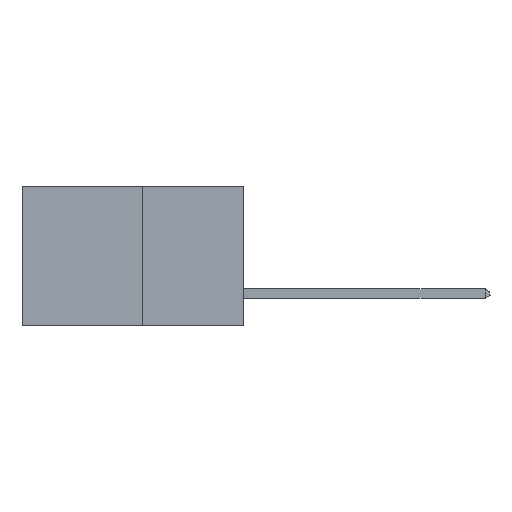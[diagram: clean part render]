
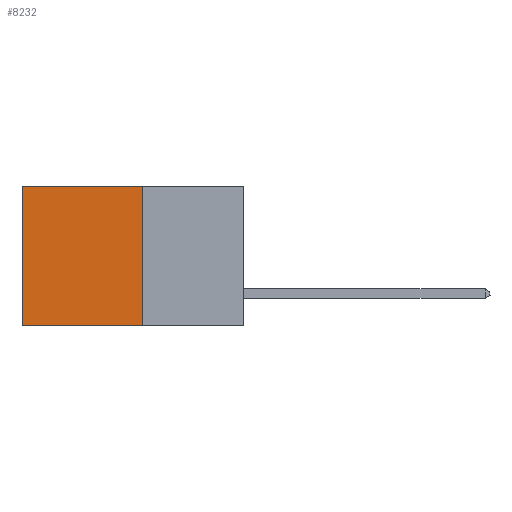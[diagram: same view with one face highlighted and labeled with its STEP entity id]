
A CAD part, left-side view. The second image highlights one B-rep face of the part: STEP entity #8232.
In plain terms, the highlighted planar face has unit normal (-1, 0, 0).
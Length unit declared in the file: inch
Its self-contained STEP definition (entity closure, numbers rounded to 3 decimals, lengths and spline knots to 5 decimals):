
#179 = LINE ( 'NONE', #2018, #6119 ) ;
#204 = FACE_OUTER_BOUND ( 'NONE', #8786, .T. ) ;
#491 = VECTOR ( 'NONE', #4156, 39.37008 ) ;
#541 = ORIENTED_EDGE ( 'NONE', *, *, #12703, .T. ) ;
#869 = ORIENTED_EDGE ( 'NONE', *, *, #9110, .T. ) ;
#2018 = CARTESIAN_POINT ( 'NONE',  ( 0.277, 0.27, 0. ) ) ;
#2374 = VECTOR ( 'NONE', #12583, 39.37008 ) ;
#3217 = CARTESIAN_POINT ( 'NONE',  ( 0.277, 0.59, 0. ) ) ;
#3485 = CARTESIAN_POINT ( 'NONE',  ( 0.277, 0.27, 0. ) ) ;
#3662 = VERTEX_POINT ( 'NONE', #4995 ) ;
#4156 = DIRECTION ( 'NONE',  ( 0., 0., -1. ) ) ;
#4217 = DIRECTION ( 'NONE',  ( 0., 1., 0. ) ) ;
#4661 = AXIS2_PLACEMENT_3D ( 'NONE', #8476, #8175, #8158 ) ;
#4995 = CARTESIAN_POINT ( 'NONE',  ( 0.277, 0.27, -0.37 ) ) ;
#5011 = ORIENTED_EDGE ( 'NONE', *, *, #7731, .F. ) ;
#5369 = LINE ( 'NONE', #7402, #2374 ) ;
#6119 = VECTOR ( 'NONE', #4217, 39.37008 ) ;
#7402 = CARTESIAN_POINT ( 'NONE',  ( 0.277, 0.27, -0.37 ) ) ;
#7562 = LINE ( 'NONE', #13592, #12735 ) ;
#7618 = VERTEX_POINT ( 'NONE', #3217 ) ;
#7731 = EDGE_CURVE ( 'NONE', #12972, #3662, #7562, .T. ) ;
#8158 = DIRECTION ( 'NONE',  ( 0., 0., -1. ) ) ;
#8175 = DIRECTION ( 'NONE',  ( 1., 0., 0. ) ) ;
#8232 = ADVANCED_FACE ( 'NONE', ( #204 ), #8440, .F. ) ;
#8440 = PLANE ( 'NONE',  #4661 ) ;
#8476 = CARTESIAN_POINT ( 'NONE',  ( 0.277, 0.27, -0.37 ) ) ;
#8786 = EDGE_LOOP ( 'NONE', ( #541, #12832, #5011, #869 ) ) ;
#8995 = LINE ( 'NONE', #10750, #491 ) ;
#9105 = VERTEX_POINT ( 'NONE', #13734 ) ;
#9110 = EDGE_CURVE ( 'NONE', #12972, #7618, #179, .T. ) ;
#10750 = CARTESIAN_POINT ( 'NONE',  ( 0.277, 0.59, -0.37 ) ) ;
#11145 = EDGE_CURVE ( 'NONE', #3662, #9105, #5369, .T. ) ;
#12583 = DIRECTION ( 'NONE',  ( 0., 1., 0. ) ) ;
#12703 = EDGE_CURVE ( 'NONE', #7618, #9105, #8995, .T. ) ;
#12735 = VECTOR ( 'NONE', #13489, 39.37008 ) ;
#12832 = ORIENTED_EDGE ( 'NONE', *, *, #11145, .F. ) ;
#12972 = VERTEX_POINT ( 'NONE', #3485 ) ;
#13489 = DIRECTION ( 'NONE',  ( 0., 0., -1. ) ) ;
#13592 = CARTESIAN_POINT ( 'NONE',  ( 0.277, 0.27, -0.37 ) ) ;
#13734 = CARTESIAN_POINT ( 'NONE',  ( 0.277, 0.59, -0.37 ) ) ;
